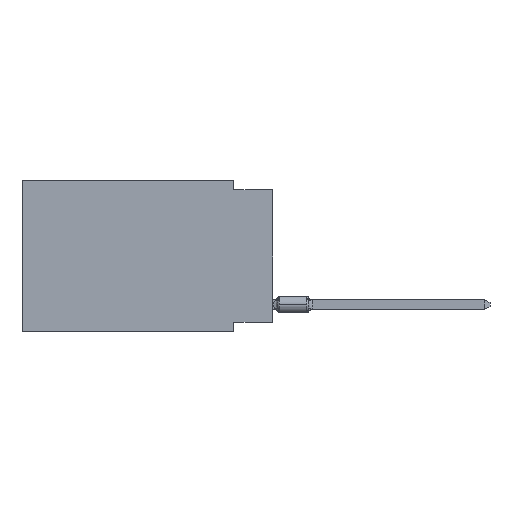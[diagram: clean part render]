
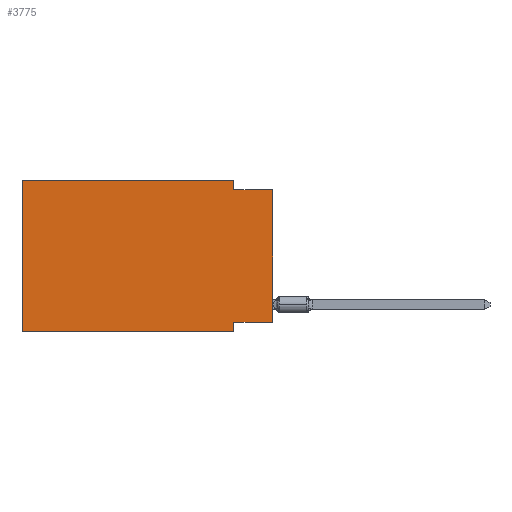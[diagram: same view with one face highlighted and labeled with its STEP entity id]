
A CAD part, left-side view. The second image highlights one B-rep face of the part: STEP entity #3775.
In plain terms, the highlighted planar face has unit normal (-1, 0, 0).
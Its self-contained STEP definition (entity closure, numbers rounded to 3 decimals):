
#457 = ORIENTED_EDGE ( 'NONE', *, *, #23823, .F. ) ;
#1492 = CARTESIAN_POINT ( 'NONE',  ( 0., 0., -9.271 ) ) ;
#1728 = EDGE_CURVE ( 'NONE', #18020, #4424, #14664, .T. ) ;
#2815 = VECTOR ( 'NONE', #22804, 1000. ) ;
#3294 = DIRECTION ( 'NONE',  ( 0., -1., 0. ) ) ;
#3388 = VERTEX_POINT ( 'NONE', #10708 ) ;
#3620 = CARTESIAN_POINT ( 'NONE',  ( 0., 16.383, -9.906 ) ) ;
#3775 = ADVANCED_FACE ( 'NONE', ( #8591 ), #4008, .F. ) ;
#3858 = CARTESIAN_POINT ( 'NONE',  ( 0., 0., -0.635 ) ) ;
#4008 = PLANE ( 'NONE',  #25839 ) ;
#4424 = VERTEX_POINT ( 'NONE', #15648 ) ;
#4739 = CARTESIAN_POINT ( 'NONE',  ( 0., 2.54, -9.906 ) ) ;
#5324 = ORIENTED_EDGE ( 'NONE', *, *, #5423, .F. ) ;
#5423 = EDGE_CURVE ( 'NONE', #23508, #19060, #8093, .T. ) ;
#5789 = DIRECTION ( 'NONE',  ( 0., 1., 0. ) ) ;
#6049 = CARTESIAN_POINT ( 'NONE',  ( 0., 0., -0.635 ) ) ;
#6258 = EDGE_CURVE ( 'NONE', #3388, #19909, #26281, .T. ) ;
#6280 = CARTESIAN_POINT ( 'NONE',  ( 0., 16.383, 0. ) ) ;
#6540 = DIRECTION ( 'NONE',  ( 0., 0., -1. ) ) ;
#7402 = VECTOR ( 'NONE', #5789, 1000. ) ;
#7431 = CARTESIAN_POINT ( 'NONE',  ( 0., 16.383, -9.906 ) ) ;
#7580 = LINE ( 'NONE', #7431, #24354 ) ;
#8093 = LINE ( 'NONE', #17089, #28311 ) ;
#8534 = ORIENTED_EDGE ( 'NONE', *, *, #6258, .F. ) ;
#8591 = FACE_OUTER_BOUND ( 'NONE', #16643, .T. ) ;
#9531 = EDGE_CURVE ( 'NONE', #16722, #23508, #15076, .T. ) ;
#10708 = CARTESIAN_POINT ( 'NONE',  ( 0., 2.54, -0.635 ) ) ;
#12336 = DIRECTION ( 'NONE',  ( 1., 0., 0. ) ) ;
#12576 = ORIENTED_EDGE ( 'NONE', *, *, #13384, .T. ) ;
#12914 = DIRECTION ( 'NONE',  ( 0., 0., 1. ) ) ;
#13384 = EDGE_CURVE ( 'NONE', #23702, #19060, #7580, .T. ) ;
#14308 = CARTESIAN_POINT ( 'NONE',  ( 0., 0., 0. ) ) ;
#14597 = ORIENTED_EDGE ( 'NONE', *, *, #27232, .F. ) ;
#14664 = LINE ( 'NONE', #23236, #21142 ) ;
#15054 = DIRECTION ( 'NONE',  ( 0., -1., 0. ) ) ;
#15076 = LINE ( 'NONE', #1492, #7402 ) ;
#15437 = DIRECTION ( 'NONE',  ( 0., 0., 1. ) ) ;
#15648 = CARTESIAN_POINT ( 'NONE',  ( 0., 2.54, 0. ) ) ;
#15903 = ORIENTED_EDGE ( 'NONE', *, *, #1728, .F. ) ;
#16643 = EDGE_LOOP ( 'NONE', ( #24708, #8534, #457, #15903, #14597, #12576, #5324, #20849 ) ) ;
#16722 = VERTEX_POINT ( 'NONE', #28665 ) ;
#17089 = CARTESIAN_POINT ( 'NONE',  ( 0., 2.54, -9.906 ) ) ;
#17221 = VECTOR ( 'NONE', #15054, 1000. ) ;
#18020 = VERTEX_POINT ( 'NONE', #28895 ) ;
#18649 = DIRECTION ( 'NONE',  ( 0., -1., 0. ) ) ;
#19060 = VERTEX_POINT ( 'NONE', #4739 ) ;
#19822 = CARTESIAN_POINT ( 'NONE',  ( 0., 16.383, 0. ) ) ;
#19909 = VERTEX_POINT ( 'NONE', #3858 ) ;
#20849 = ORIENTED_EDGE ( 'NONE', *, *, #9531, .F. ) ;
#21142 = VECTOR ( 'NONE', #3294, 1000. ) ;
#21663 = DIRECTION ( 'NONE',  ( 0., 0., -1. ) ) ;
#22804 = DIRECTION ( 'NONE',  ( 0., 0., -1. ) ) ;
#23236 = CARTESIAN_POINT ( 'NONE',  ( 0., 16.383, 0. ) ) ;
#23508 = VERTEX_POINT ( 'NONE', #28800 ) ;
#23702 = VERTEX_POINT ( 'NONE', #3620 ) ;
#23823 = EDGE_CURVE ( 'NONE', #4424, #3388, #26808, .T. ) ;
#24288 = LINE ( 'NONE', #6280, #29064 ) ;
#24337 = VECTOR ( 'NONE', #12914, 1000. ) ;
#24354 = VECTOR ( 'NONE', #18649, 1000. ) ;
#24708 = ORIENTED_EDGE ( 'NONE', *, *, #25515, .T. ) ;
#25017 = CARTESIAN_POINT ( 'NONE',  ( 0., 2.54, 0. ) ) ;
#25515 = EDGE_CURVE ( 'NONE', #16722, #19909, #25543, .T. ) ;
#25543 = LINE ( 'NONE', #14308, #24337 ) ;
#25839 = AXIS2_PLACEMENT_3D ( 'NONE', #19822, #12336, #6540 ) ;
#26281 = LINE ( 'NONE', #6049, #17221 ) ;
#26808 = LINE ( 'NONE', #25017, #2815 ) ;
#27232 = EDGE_CURVE ( 'NONE', #23702, #18020, #24288, .T. ) ;
#28311 = VECTOR ( 'NONE', #21663, 1000. ) ;
#28665 = CARTESIAN_POINT ( 'NONE',  ( 0., 0., -9.271 ) ) ;
#28800 = CARTESIAN_POINT ( 'NONE',  ( 0., 2.54, -9.271 ) ) ;
#28895 = CARTESIAN_POINT ( 'NONE',  ( 0., 16.383, 0. ) ) ;
#29064 = VECTOR ( 'NONE', #15437, 1000. ) ;
